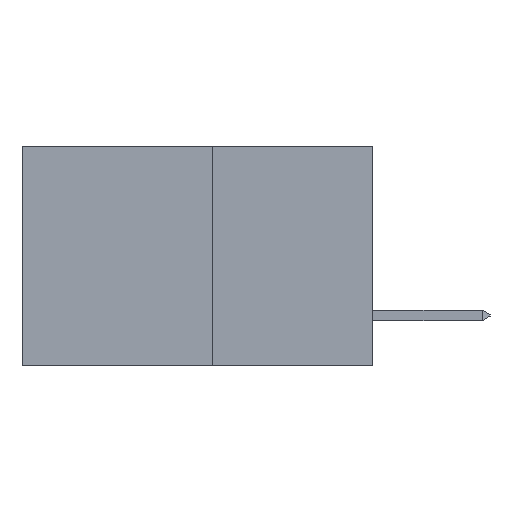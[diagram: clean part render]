
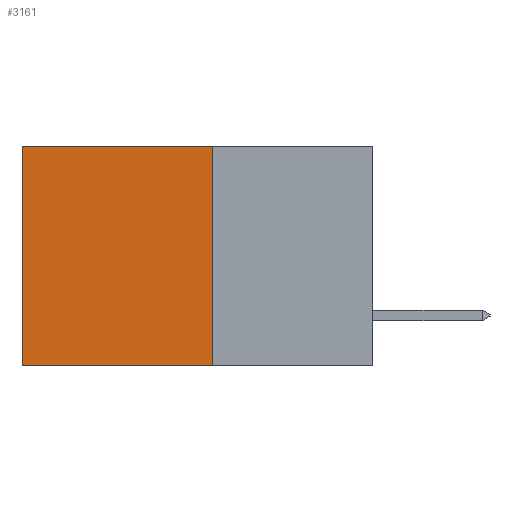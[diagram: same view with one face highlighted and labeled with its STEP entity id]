
A CAD part, left-side view. The second image highlights one B-rep face of the part: STEP entity #3161.
In plain terms, the highlighted planar face has unit normal (-1, 0, 0).
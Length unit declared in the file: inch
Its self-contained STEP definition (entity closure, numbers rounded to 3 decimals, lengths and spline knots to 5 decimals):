
#284 = LINE ( 'NONE', #4886, #5533 ) ;
#404 = DIRECTION ( 'NONE',  ( 0., 0., -1. ) ) ;
#552 = DIRECTION ( 'NONE',  ( 0., 0., -1. ) ) ;
#599 = CARTESIAN_POINT ( 'NONE',  ( 0.277, 0.59, -0.37 ) ) ;
#1101 = CARTESIAN_POINT ( 'NONE',  ( 0.277, 0.27, -0.37 ) ) ;
#1207 = ORIENTED_EDGE ( 'NONE', *, *, #2377, .F. ) ;
#1445 = DIRECTION ( 'NONE',  ( 0., 0., -1. ) ) ;
#1637 = EDGE_CURVE ( 'NONE', #6734, #2650, #5860, .T. ) ;
#1688 = DIRECTION ( 'NONE',  ( 1., 0., 0. ) ) ;
#1737 = VERTEX_POINT ( 'NONE', #11030 ) ;
#2377 = EDGE_CURVE ( 'NONE', #10300, #6734, #5391, .T. ) ;
#2633 = DIRECTION ( 'NONE',  ( 0., 1., 0. ) ) ;
#2650 = VERTEX_POINT ( 'NONE', #9133 ) ;
#2668 = CARTESIAN_POINT ( 'NONE',  ( 0.277, 0.27, -0.37 ) ) ;
#3161 = ADVANCED_FACE ( 'NONE', ( #11658 ), #11248, .F. ) ;
#3868 = VECTOR ( 'NONE', #404, 39.37008 ) ;
#4361 = ORIENTED_EDGE ( 'NONE', *, *, #13098, .T. ) ;
#4886 = CARTESIAN_POINT ( 'NONE',  ( 0.277, 0.27, 0. ) ) ;
#5391 = LINE ( 'NONE', #11728, #10415 ) ;
#5533 = VECTOR ( 'NONE', #5889, 39.37008 ) ;
#5860 = LINE ( 'NONE', #2668, #10913 ) ;
#5889 = DIRECTION ( 'NONE',  ( 0., 1., 0. ) ) ;
#6734 = VERTEX_POINT ( 'NONE', #1101 ) ;
#6808 = EDGE_CURVE ( 'NONE', #1737, #2650, #11788, .T. ) ;
#7250 = EDGE_LOOP ( 'NONE', ( #8141, #11129, #1207, #4361 ) ) ;
#7502 = AXIS2_PLACEMENT_3D ( 'NONE', #11354, #1688, #1445 ) ;
#8141 = ORIENTED_EDGE ( 'NONE', *, *, #6808, .T. ) ;
#9133 = CARTESIAN_POINT ( 'NONE',  ( 0.277, 0.59, -0.37 ) ) ;
#10300 = VERTEX_POINT ( 'NONE', #11024 ) ;
#10415 = VECTOR ( 'NONE', #552, 39.37008 ) ;
#10913 = VECTOR ( 'NONE', #2633, 39.37008 ) ;
#11024 = CARTESIAN_POINT ( 'NONE',  ( 0.277, 0.27, 0. ) ) ;
#11030 = CARTESIAN_POINT ( 'NONE',  ( 0.277, 0.59, 0. ) ) ;
#11129 = ORIENTED_EDGE ( 'NONE', *, *, #1637, .F. ) ;
#11248 = PLANE ( 'NONE',  #7502 ) ;
#11354 = CARTESIAN_POINT ( 'NONE',  ( 0.277, 0.27, -0.37 ) ) ;
#11658 = FACE_OUTER_BOUND ( 'NONE', #7250, .T. ) ;
#11728 = CARTESIAN_POINT ( 'NONE',  ( 0.277, 0.27, -0.37 ) ) ;
#11788 = LINE ( 'NONE', #599, #3868 ) ;
#13098 = EDGE_CURVE ( 'NONE', #10300, #1737, #284, .T. ) ;
